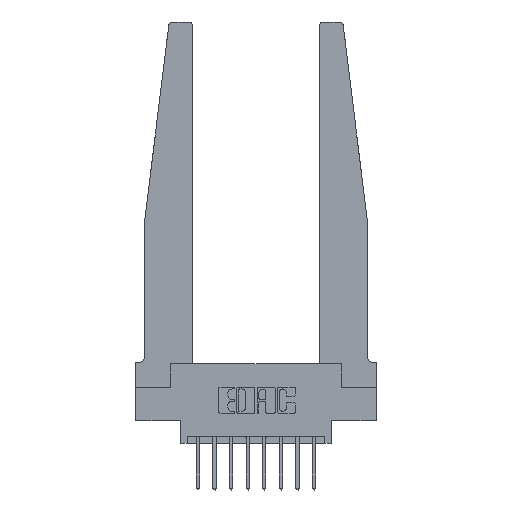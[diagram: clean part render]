
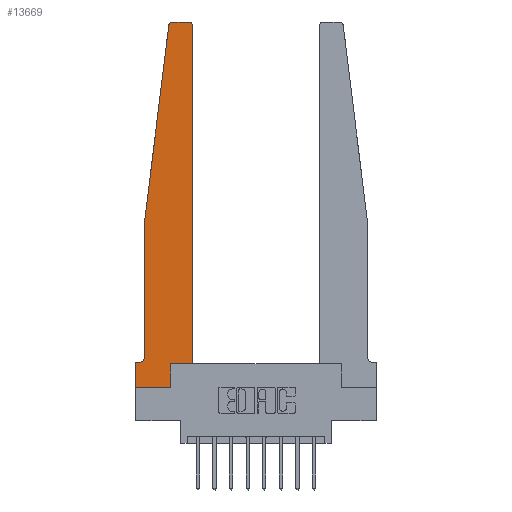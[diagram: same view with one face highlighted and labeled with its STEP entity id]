
A CAD part, top view. The second image highlights one B-rep face of the part: STEP entity #13669.
In plain terms, the highlighted planar face has unit normal (0, 0, 1).
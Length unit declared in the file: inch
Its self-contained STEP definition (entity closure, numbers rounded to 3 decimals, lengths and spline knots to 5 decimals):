
#10 = DIRECTION ( 'NONE',  ( 0., 0., 1. ) ) ;
#77 = DIRECTION ( 'NONE',  ( 0., 1., 0. ) ) ;
#129 = FACE_OUTER_BOUND ( 'NONE', #10552, .T. ) ;
#203 = DIRECTION ( 'NONE',  ( 1., 0., 0. ) ) ;
#285 = EDGE_CURVE ( 'NONE', #7689, #12178, #13896, .T. ) ;
#484 = ORIENTED_EDGE ( 'NONE', *, *, #13172, .T. ) ;
#834 = CARTESIAN_POINT ( 'NONE',  ( 0.27653, 2.75, 0.37 ) ) ;
#856 = ORIENTED_EDGE ( 'NONE', *, *, #7625, .T. ) ;
#887 = LINE ( 'NONE', #5342, #3584 ) ;
#915 = DIRECTION ( 'NONE',  ( 0., 1., 0. ) ) ;
#1168 = VERTEX_POINT ( 'NONE', #3475 ) ;
#1218 = CIRCLE ( 'NONE', #3255, 0.03 ) ;
#1224 = EDGE_CURVE ( 'NONE', #6326, #13762, #887, .T. ) ;
#1341 = VERTEX_POINT ( 'NONE', #11789 ) ;
#1577 = ORIENTED_EDGE ( 'NONE', *, *, #1224, .T. ) ;
#1949 = ORIENTED_EDGE ( 'NONE', *, *, #8008, .T. ) ;
#2487 = PLANE ( 'NONE',  #13888 ) ;
#2515 = LINE ( 'NONE', #7743, #2879 ) ;
#2591 = CARTESIAN_POINT ( 'NONE',  ( 0.24675, 2.72367, 0.37 ) ) ;
#2620 = DIRECTION ( 'NONE',  ( 1., 0., 0. ) ) ;
#2705 = VERTEX_POINT ( 'NONE', #9970 ) ;
#2879 = VECTOR ( 'NONE', #915, 39.37008 ) ;
#2893 = CARTESIAN_POINT ( 'NONE',  ( 0.2605, 0., 0.37 ) ) ;
#3255 = AXIS2_PLACEMENT_3D ( 'NONE', #6869, #10, #8002 ) ;
#3475 = CARTESIAN_POINT ( 'NONE',  ( 0., 0.1875, 0.37 ) ) ;
#3584 = VECTOR ( 'NONE', #77, 39.37008 ) ;
#3848 = VERTEX_POINT ( 'NONE', #5341 ) ;
#3850 = EDGE_CURVE ( 'NONE', #3848, #4160, #11140, .T. ) ;
#4160 = VERTEX_POINT ( 'NONE', #834 ) ;
#4182 = CARTESIAN_POINT ( 'NONE',  ( 0.015, 0.2375, 0.37 ) ) ;
#4213 = CARTESIAN_POINT ( 'NONE',  ( 0.25, 2.75, 0.37 ) ) ;
#4559 = VERTEX_POINT ( 'NONE', #2591 ) ;
#4596 = CARTESIAN_POINT ( 'NONE',  ( 0.425, 0.18, 0.37 ) ) ;
#4645 = LINE ( 'NONE', #11809, #9944 ) ;
#4840 = CARTESIAN_POINT ( 'NONE',  ( 0., 0., 0.37 ) ) ;
#4865 = VECTOR ( 'NONE', #9668, 39.37008 ) ;
#4986 = DIRECTION ( 'NONE',  ( 1., 0., 0. ) ) ;
#5060 = DIRECTION ( 'NONE',  ( -0.122, -0.992, 0. ) ) ;
#5318 = DIRECTION ( 'NONE',  ( -1., 0., 0. ) ) ;
#5341 = CARTESIAN_POINT ( 'NONE',  ( 0.395, 2.75, 0.37 ) ) ;
#5342 = CARTESIAN_POINT ( 'NONE',  ( 0.2605, 0.18, 0.37 ) ) ;
#5586 = AXIS2_PLACEMENT_3D ( 'NONE', #6752, #14658, #7884 ) ;
#5924 = CARTESIAN_POINT ( 'NONE',  ( 0., 0.1875, 0.37 ) ) ;
#6270 = VERTEX_POINT ( 'NONE', #7367 ) ;
#6271 = VECTOR ( 'NONE', #5060, 39.37008 ) ;
#6326 = VERTEX_POINT ( 'NONE', #2893 ) ;
#6451 = LINE ( 'NONE', #9430, #12113 ) ;
#6752 = CARTESIAN_POINT ( 'NONE',  ( 0.27653, 2.72, 0.37 ) ) ;
#6869 = CARTESIAN_POINT ( 'NONE',  ( 0.395, 2.72, 0.37 ) ) ;
#7063 = DIRECTION ( 'NONE',  ( 0., 0., 1. ) ) ;
#7367 = CARTESIAN_POINT ( 'NONE',  ( 0., 0., 0.37 ) ) ;
#7625 = EDGE_CURVE ( 'NONE', #1168, #6270, #10505, .T. ) ;
#7645 = ORIENTED_EDGE ( 'NONE', *, *, #9432, .T. ) ;
#7689 = VERTEX_POINT ( 'NONE', #11721 ) ;
#7743 = CARTESIAN_POINT ( 'NONE',  ( 0.425, 0.18, 0.37 ) ) ;
#7884 = DIRECTION ( 'NONE',  ( 1., 0., 0. ) ) ;
#8002 = DIRECTION ( 'NONE',  ( 1., 0., 0. ) ) ;
#8008 = EDGE_CURVE ( 'NONE', #14070, #2705, #2515, .T. ) ;
#8077 = EDGE_CURVE ( 'NONE', #4160, #4559, #13537, .T. ) ;
#8135 = VECTOR ( 'NONE', #13277, 39.37008 ) ;
#8529 = ORIENTED_EDGE ( 'NONE', *, *, #285, .T. ) ;
#8922 = AXIS2_PLACEMENT_3D ( 'NONE', #4182, #12090, #5318 ) ;
#9430 = CARTESIAN_POINT ( 'NONE',  ( 0., 0., 0.37 ) ) ;
#9432 = EDGE_CURVE ( 'NONE', #13762, #14070, #4645, .T. ) ;
#9486 = CARTESIAN_POINT ( 'NONE',  ( 0.2605, 0.18, 0.37 ) ) ;
#9564 = CARTESIAN_POINT ( 'NONE',  ( 0.065, 0.2375, 0.37 ) ) ;
#9668 = DIRECTION ( 'NONE',  ( 0., -1., 0. ) ) ;
#9944 = VECTOR ( 'NONE', #4986, 39.37008 ) ;
#9970 = CARTESIAN_POINT ( 'NONE',  ( 0.425, 2.72, 0.37 ) ) ;
#10429 = EDGE_CURVE ( 'NONE', #12178, #1341, #13303, .T. ) ;
#10505 = LINE ( 'NONE', #4840, #13551 ) ;
#10552 = EDGE_LOOP ( 'NONE', ( #13500, #13844, #14183, #8529, #11883, #484, #856, #12964, #1577, #7645, #1949, #11003 ) ) ;
#10628 = CARTESIAN_POINT ( 'NONE',  ( 0.065, 0.1875, 0.37 ) ) ;
#10687 = CARTESIAN_POINT ( 'NONE',  ( 0.065, 1.25, 0.37 ) ) ;
#10741 = CARTESIAN_POINT ( 'NONE',  ( 0.065, 1.25, 0.37 ) ) ;
#11003 = ORIENTED_EDGE ( 'NONE', *, *, #13580, .T. ) ;
#11140 = LINE ( 'NONE', #4213, #8135 ) ;
#11622 = DIRECTION ( 'NONE',  ( 0., -1., 0. ) ) ;
#11721 = CARTESIAN_POINT ( 'NONE',  ( 0.065, 1.25, 0.37 ) ) ;
#11780 = DIRECTION ( 'NONE',  ( -1., 0., 0. ) ) ;
#11789 = CARTESIAN_POINT ( 'NONE',  ( 0.015, 0.1875, 0.37 ) ) ;
#11809 = CARTESIAN_POINT ( 'NONE',  ( 0.425, 0.18, 0.37 ) ) ;
#11883 = ORIENTED_EDGE ( 'NONE', *, *, #10429, .T. ) ;
#12090 = DIRECTION ( 'NONE',  ( 0., 0., -1. ) ) ;
#12113 = VECTOR ( 'NONE', #2620, 39.37008 ) ;
#12178 = VERTEX_POINT ( 'NONE', #9564 ) ;
#12182 = EDGE_CURVE ( 'NONE', #4559, #7689, #12294, .T. ) ;
#12269 = VECTOR ( 'NONE', #11780, 39.37008 ) ;
#12294 = LINE ( 'NONE', #10687, #6271 ) ;
#12457 = EDGE_CURVE ( 'NONE', #6270, #6326, #6451, .T. ) ;
#12615 = LINE ( 'NONE', #10628, #12269 ) ;
#12964 = ORIENTED_EDGE ( 'NONE', *, *, #12457, .T. ) ;
#13172 = EDGE_CURVE ( 'NONE', #1341, #1168, #12615, .T. ) ;
#13277 = DIRECTION ( 'NONE',  ( -1., 0., 0. ) ) ;
#13303 = CIRCLE ( 'NONE', #8922, 0.05 ) ;
#13500 = ORIENTED_EDGE ( 'NONE', *, *, #3850, .T. ) ;
#13537 = CIRCLE ( 'NONE', #5586, 0.03 ) ;
#13551 = VECTOR ( 'NONE', #11622, 39.37008 ) ;
#13580 = EDGE_CURVE ( 'NONE', #2705, #3848, #1218, .T. ) ;
#13669 = ADVANCED_FACE ( 'NONE', ( #129 ), #2487, .T. ) ;
#13762 = VERTEX_POINT ( 'NONE', #9486 ) ;
#13844 = ORIENTED_EDGE ( 'NONE', *, *, #8077, .T. ) ;
#13888 = AXIS2_PLACEMENT_3D ( 'NONE', #5924, #7063, #203 ) ;
#13896 = LINE ( 'NONE', #10741, #4865 ) ;
#14070 = VERTEX_POINT ( 'NONE', #4596 ) ;
#14183 = ORIENTED_EDGE ( 'NONE', *, *, #12182, .T. ) ;
#14658 = DIRECTION ( 'NONE',  ( 0., 0., 1. ) ) ;
